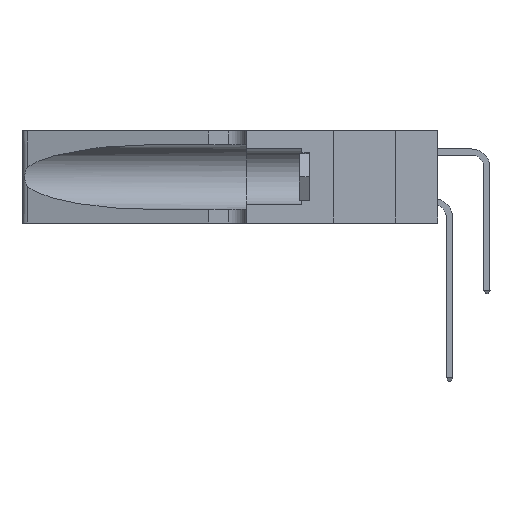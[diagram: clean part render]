
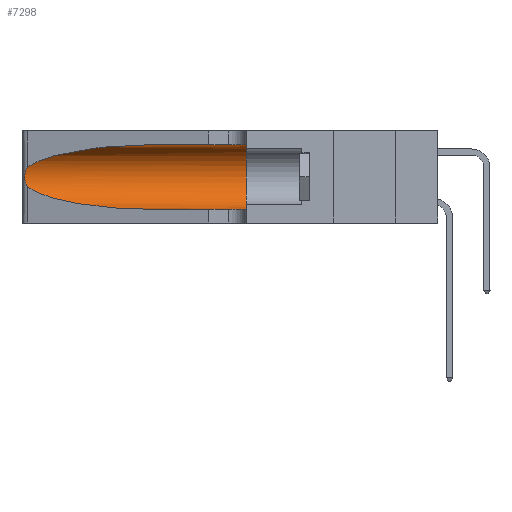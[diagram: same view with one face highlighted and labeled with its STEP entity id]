
A CAD part, left-side view. The second image highlights one B-rep face of the part: STEP entity #7298.
In plain terms, the highlighted cylindrical face has radius 3.308 mm (diameter 6.617 mm), a partial arc.
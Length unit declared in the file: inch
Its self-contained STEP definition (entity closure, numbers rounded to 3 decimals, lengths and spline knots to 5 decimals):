
#417 = CARTESIAN_POINT ( 'NONE',  ( 0.26075, 1.23896, 0.178 ) ) ;
#1094 = DIRECTION ( 'NONE',  ( 0., -1., 0. ) ) ;
#1514 = VECTOR ( 'NONE', #1094, 39.37008 ) ;
#1827 = CYLINDRICAL_SURFACE ( 'NONE', #21464, 0.13025 ) ;
#2782 = FACE_OUTER_BOUND ( 'NONE', #24879, .T. ) ;
#3503 = CARTESIAN_POINT ( 'NONE',  ( 0.25856, 1.23593, 0.16098 ) ) ;
#3806 = CARTESIAN_POINT ( 'NONE',  ( 0.25487, 1.22718, 0.22369 ) ) ;
#4410 = CIRCLE ( 'NONE', #4969, 0.13025 ) ;
#4608 = CARTESIAN_POINT ( 'NONE',  ( 0.1305, 0.35, 0.31525 ) ) ;
#4776 = B_SPLINE_CURVE_WITH_KNOTS ( 'NONE', 3,
 ( #30918, #24832, #9578, #33967, #15754, #36981, #18856, #417, #21892, #3503, #24974, #6598, #27984, #9705 ),
 .UNSPECIFIED., .F., .F.,
 ( 4, 2, 2, 2, 2, 2, 4 ),
 ( 0., 0.00027, 0.00053, 0.00107, 0.0016, 0.00187, 0.00214 ),
 .UNSPECIFIED. ) ;
#4894 = CARTESIAN_POINT ( 'NONE',  ( 0.18966, 0.96281, 0.05475 ) ) ;
#4969 = AXIS2_PLACEMENT_3D ( 'NONE', #7041, #28408, #10155 ) ;
#6598 = CARTESIAN_POINT ( 'NONE',  ( 0.25639, 1.23186, 0.15144 ) ) ;
#7041 = CARTESIAN_POINT ( 'NONE',  ( 0.1305, 0.35, 0.185 ) ) ;
#7149 = EDGE_CURVE ( 'NONE', #23342, #22537, #17894, .T. ) ;
#7298 = ADVANCED_FACE ( 'NONE', ( #2782 ), #1827, .F. ) ;
#7899 = CARTESIAN_POINT ( 'NONE',  ( 0.25487, 1.22718, 0.14631 ) ) ;
#8966 = ORIENTED_EDGE ( 'NONE', *, *, #15728, .T. ) ;
#9430 = CARTESIAN_POINT ( 'NONE',  ( 0.1305, 0.72297, 0.31525 ) ) ;
#9578 = CARTESIAN_POINT ( 'NONE',  ( 0.25639, 1.23184, 0.21858 ) ) ;
#9705 = CARTESIAN_POINT ( 'NONE',  ( 0.25487, 1.22718, 0.14631 ) ) ;
#9923 = ORIENTED_EDGE ( 'NONE', *, *, #31386, .T. ) ;
#10155 = DIRECTION ( 'NONE',  ( 0., 0., 1. ) ) ;
#12537 = CARTESIAN_POINT ( 'NONE',  ( 0.18966, 0.96281, 0.31525 ) ) ;
#12904 = DIRECTION ( 'NONE',  ( 0., -1., 0. ) ) ;
#14007 = EDGE_CURVE ( 'NONE', #38409, #32715, #4776, .T. ) ;
#14069 = CARTESIAN_POINT ( 'NONE',  ( 0.2373, 1.15595, 0.08982 ) ) ;
#15610 = CARTESIAN_POINT ( 'NONE',  ( 0.25487, 1.22718, 0.22369 ) ) ;
#15728 = EDGE_CURVE ( 'NONE', #23342, #38409, #19575, .T. ) ;
#15754 = CARTESIAN_POINT ( 'NONE',  ( 0.25854, 1.2359, 0.20912 ) ) ;
#16244 = VERTEX_POINT ( 'NONE', #36684 ) ;
#16452 = CARTESIAN_POINT ( 'NONE',  ( 0.1305, 1.61858, 0.31525 ) ) ;
#17894 = LINE ( 'NONE', #16452, #1514 ) ;
#18856 = CARTESIAN_POINT ( 'NONE',  ( 0.26075, 1.23896, 0.19203 ) ) ;
#19575 =( BOUNDED_CURVE ( )  B_SPLINE_CURVE ( 3, ( #9430, #12537, #33818, #15610 ),
 .UNSPECIFIED., .F., .F. ) 
 B_SPLINE_CURVE_WITH_KNOTS ( ( 4, 4 ),
 ( 1.5708, 2.84003 ),
 .UNSPECIFIED. ) 
 CURVE ( )  GEOMETRIC_REPRESENTATION_ITEM ( )  RATIONAL_B_SPLINE_CURVE ( ( 1., 0.87, 0.87, 1. ) ) 
 REPRESENTATION_ITEM ( '' )  );
#19921 = LINE ( 'NONE', #31131, #36047 ) ;
#20170 = DIRECTION ( 'NONE',  ( 0., 0., -1. ) ) ;
#20405 = CARTESIAN_POINT ( 'NONE',  ( 0.1305, 0.72297, 0.31525 ) ) ;
#21464 = AXIS2_PLACEMENT_3D ( 'NONE', #32247, #38313, #20170 ) ;
#21892 = CARTESIAN_POINT ( 'NONE',  ( 0.26017, 1.23833, 0.17102 ) ) ;
#22387 = EDGE_CURVE ( 'NONE', #22537, #16244, #4410, .T. ) ;
#22537 = VERTEX_POINT ( 'NONE', #4608 ) ;
#23342 = VERTEX_POINT ( 'NONE', #20405 ) ;
#24832 = CARTESIAN_POINT ( 'NONE',  ( 0.25555, 1.22994, 0.2215 ) ) ;
#24879 = EDGE_LOOP ( 'NONE', ( #8966, #33300, #9923, #27125, #36131, #29974 ) ) ;
#24974 = CARTESIAN_POINT ( 'NONE',  ( 0.25789, 1.23486, 0.15765 ) ) ;
#26322 = CARTESIAN_POINT ( 'NONE',  ( 0.1305, 0.72297, 0.05475 ) ) ;
#27125 = ORIENTED_EDGE ( 'NONE', *, *, #32422, .T. ) ;
#27984 = CARTESIAN_POINT ( 'NONE',  ( 0.25555, 1.22993, 0.14849 ) ) ;
#28408 = DIRECTION ( 'NONE',  ( 0., 1., 0. ) ) ;
#29974 = ORIENTED_EDGE ( 'NONE', *, *, #7149, .F. ) ;
#30918 = CARTESIAN_POINT ( 'NONE',  ( 0.25487, 1.22718, 0.22369 ) ) ;
#31131 = CARTESIAN_POINT ( 'NONE',  ( 0.1305, 1.61858, 0.05475 ) ) ;
#31386 = EDGE_CURVE ( 'NONE', #32715, #37848, #38537, .T. ) ;
#32054 = CARTESIAN_POINT ( 'NONE',  ( 0.1305, 0.72297, 0.05475 ) ) ;
#32247 = CARTESIAN_POINT ( 'NONE',  ( 0.1305, 1.61858, 0.185 ) ) ;
#32422 = EDGE_CURVE ( 'NONE', #37848, #16244, #19921, .T. ) ;
#32715 = VERTEX_POINT ( 'NONE', #7899 ) ;
#33300 = ORIENTED_EDGE ( 'NONE', *, *, #14007, .T. ) ;
#33818 = CARTESIAN_POINT ( 'NONE',  ( 0.2373, 1.15595, 0.28018 ) ) ;
#33967 = CARTESIAN_POINT ( 'NONE',  ( 0.25787, 1.23484, 0.2124 ) ) ;
#35320 = CARTESIAN_POINT ( 'NONE',  ( 0.25487, 1.22718, 0.14631 ) ) ;
#36047 = VECTOR ( 'NONE', #12904, 39.37008 ) ;
#36131 = ORIENTED_EDGE ( 'NONE', *, *, #22387, .F. ) ;
#36684 = CARTESIAN_POINT ( 'NONE',  ( 0.1305, 0.35, 0.05475 ) ) ;
#36981 = CARTESIAN_POINT ( 'NONE',  ( 0.26018, 1.23835, 0.19895 ) ) ;
#37848 = VERTEX_POINT ( 'NONE', #32054 ) ;
#38313 = DIRECTION ( 'NONE',  ( 0., -1., 0. ) ) ;
#38409 = VERTEX_POINT ( 'NONE', #3806 ) ;
#38537 =( BOUNDED_CURVE ( )  B_SPLINE_CURVE ( 3, ( #35320, #14069, #4894, #26322 ),
 .UNSPECIFIED., .F., .T. ) 
 B_SPLINE_CURVE_WITH_KNOTS ( ( 4, 4 ),
 ( 3.44316, 4.71239 ),
 .UNSPECIFIED. ) 
 CURVE ( )  GEOMETRIC_REPRESENTATION_ITEM ( )  RATIONAL_B_SPLINE_CURVE ( ( 1., 0.87, 0.87, 1. ) ) 
 REPRESENTATION_ITEM ( '' )  );
